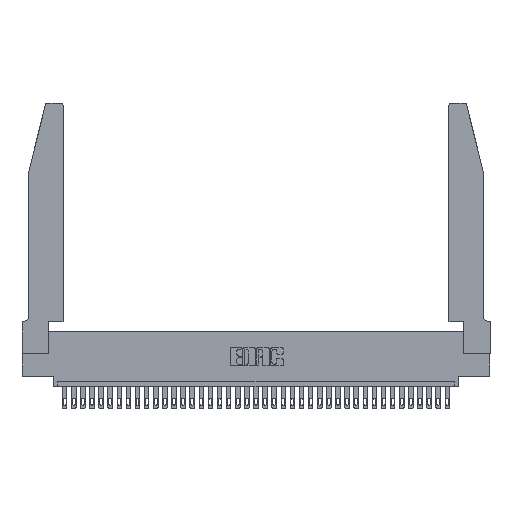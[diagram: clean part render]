
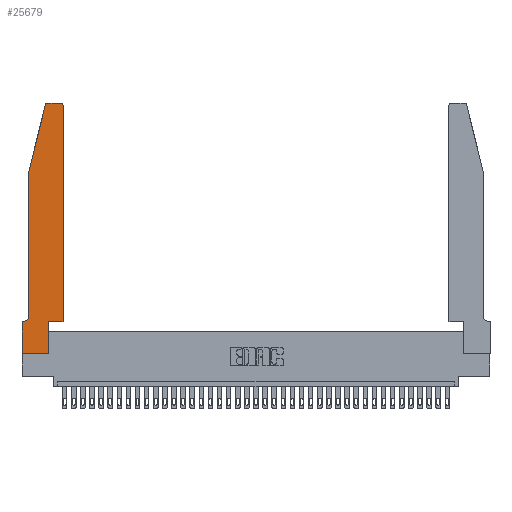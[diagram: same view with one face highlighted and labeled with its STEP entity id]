
A CAD part, top view. The second image highlights one B-rep face of the part: STEP entity #25679.
In plain terms, the highlighted planar face has unit normal (0, 0, 1).
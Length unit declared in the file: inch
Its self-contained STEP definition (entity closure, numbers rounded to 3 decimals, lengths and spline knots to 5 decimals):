
#149 = ORIENTED_EDGE ( 'NONE', *, *, #27881, .T. ) ;
#328 = VERTEX_POINT ( 'NONE', #6123 ) ;
#827 = LINE ( 'NONE', #27779, #32535 ) ;
#901 = EDGE_CURVE ( 'NONE', #5973, #25247, #16277, .T. ) ;
#1296 = CARTESIAN_POINT ( 'NONE',  ( 0., 0., 0.37 ) ) ;
#1358 = VERTEX_POINT ( 'NONE', #23213 ) ;
#1523 = CARTESIAN_POINT ( 'NONE',  ( 0.2865, 0.35, 0.37 ) ) ;
#1813 = ORIENTED_EDGE ( 'NONE', *, *, #10151, .T. ) ;
#2180 = ORIENTED_EDGE ( 'NONE', *, *, #6157, .T. ) ;
#2264 = CARTESIAN_POINT ( 'NONE',  ( 0.284, 2.72, 0.37 ) ) ;
#2333 = EDGE_CURVE ( 'NONE', #1358, #5973, #3722, .T. ) ;
#2733 = EDGE_CURVE ( 'NONE', #30739, #11146, #34075, .T. ) ;
#2929 = VERTEX_POINT ( 'NONE', #9198 ) ;
#2999 = VECTOR ( 'NONE', #15496, 39.37008 ) ;
#3722 = CIRCLE ( 'NONE', #23131, 0.07 ) ;
#3859 = FACE_OUTER_BOUND ( 'NONE', #23559, .T. ) ;
#4336 = CARTESIAN_POINT ( 'NONE',  ( 0., 0.35, 0.37 ) ) ;
#4540 = CARTESIAN_POINT ( 'NONE',  ( 0.25487, 2.72718, 0.37 ) ) ;
#4956 = CARTESIAN_POINT ( 'NONE',  ( 0.4505, 0.35, 0.37 ) ) ;
#5092 = DIRECTION ( 'NONE',  ( 1., 0., 0. ) ) ;
#5249 = LINE ( 'NONE', #1523, #2999 ) ;
#5566 = PLANE ( 'NONE',  #6493 ) ;
#5584 = VERTEX_POINT ( 'NONE', #31289 ) ;
#5973 = VERTEX_POINT ( 'NONE', #17368 ) ;
#6123 = CARTESIAN_POINT ( 'NONE',  ( 0., 0., 0.37 ) ) ;
#6157 = EDGE_CURVE ( 'NONE', #5584, #30739, #11033, .T. ) ;
#6173 = VECTOR ( 'NONE', #15835, 39.37008 ) ;
#6493 = AXIS2_PLACEMENT_3D ( 'NONE', #25360, #31089, #13894 ) ;
#6635 = DIRECTION ( 'NONE',  ( -1., 0., 0. ) ) ;
#6755 = EDGE_CURVE ( 'NONE', #11146, #10563, #12286, .T. ) ;
#7275 = EDGE_CURVE ( 'NONE', #328, #8594, #35431, .T. ) ;
#7518 = ORIENTED_EDGE ( 'NONE', *, *, #2733, .T. ) ;
#7609 = DIRECTION ( 'NONE',  ( -0.239, -0.971, 0. ) ) ;
#8113 = DIRECTION ( 'NONE',  ( 0., 0., 1. ) ) ;
#8195 = CARTESIAN_POINT ( 'NONE',  ( 0.2865, 0.35, 0.37 ) ) ;
#8306 = AXIS2_PLACEMENT_3D ( 'NONE', #16663, #22004, #5092 ) ;
#8594 = VERTEX_POINT ( 'NONE', #35665 ) ;
#9198 = CARTESIAN_POINT ( 'NONE',  ( 0.4505, 2.72, 0.37 ) ) ;
#9960 = VECTOR ( 'NONE', #32104, 39.37008 ) ;
#10151 = EDGE_CURVE ( 'NONE', #26637, #32149, #827, .T. ) ;
#10563 = VERTEX_POINT ( 'NONE', #15590 ) ;
#11033 = LINE ( 'NONE', #36269, #13682 ) ;
#11146 = VERTEX_POINT ( 'NONE', #4540 ) ;
#11243 = EDGE_CURVE ( 'NONE', #8594, #26637, #5249, .T. ) ;
#11865 = CARTESIAN_POINT ( 'NONE',  ( 0.0755, 0.35, 0.37 ) ) ;
#11964 = ORIENTED_EDGE ( 'NONE', *, *, #7275, .T. ) ;
#12286 = LINE ( 'NONE', #21658, #34613 ) ;
#12341 = CARTESIAN_POINT ( 'NONE',  ( 0.0755, 2., 0.37 ) ) ;
#12414 = ORIENTED_EDGE ( 'NONE', *, *, #2333, .T. ) ;
#12809 = CARTESIAN_POINT ( 'NONE',  ( 0.4505, 0.35, 0.37 ) ) ;
#13217 = EDGE_CURVE ( 'NONE', #10563, #1358, #33958, .T. ) ;
#13682 = VECTOR ( 'NONE', #15473, 39.37008 ) ;
#13785 = ORIENTED_EDGE ( 'NONE', *, *, #35846, .T. ) ;
#13894 = DIRECTION ( 'NONE',  ( 1., 0., 0. ) ) ;
#14136 = LINE ( 'NONE', #1296, #22592 ) ;
#15473 = DIRECTION ( 'NONE',  ( -1., 0., 0. ) ) ;
#15496 = DIRECTION ( 'NONE',  ( 0., 1., 0. ) ) ;
#15590 = CARTESIAN_POINT ( 'NONE',  ( 0.0755, 2., 0.37 ) ) ;
#15835 = DIRECTION ( 'NONE',  ( 0., -1., 0. ) ) ;
#16038 = AXIS2_PLACEMENT_3D ( 'NONE', #2264, #8113, #22303 ) ;
#16277 = LINE ( 'NONE', #11865, #31441 ) ;
#16663 = CARTESIAN_POINT ( 'NONE',  ( 0.4205, 2.72, 0.37 ) ) ;
#17368 = CARTESIAN_POINT ( 'NONE',  ( 0.0055, 0.35, 0.37 ) ) ;
#20556 = ORIENTED_EDGE ( 'NONE', *, *, #901, .T. ) ;
#20938 = EDGE_CURVE ( 'NONE', #25247, #328, #14136, .T. ) ;
#21658 = CARTESIAN_POINT ( 'NONE',  ( 0.0755, 2., 0.37 ) ) ;
#22004 = DIRECTION ( 'NONE',  ( 0., 0., 1. ) ) ;
#22303 = DIRECTION ( 'NONE',  ( 1., 0., 0. ) ) ;
#22393 = ORIENTED_EDGE ( 'NONE', *, *, #20938, .T. ) ;
#22592 = VECTOR ( 'NONE', #32202, 39.37008 ) ;
#23131 = AXIS2_PLACEMENT_3D ( 'NONE', #23674, #24041, #26917 ) ;
#23213 = CARTESIAN_POINT ( 'NONE',  ( 0.0755, 0.42, 0.37 ) ) ;
#23559 = EDGE_LOOP ( 'NONE', ( #2180, #7518, #34823, #26884, #12414, #20556, #22393, #11964, #29960, #1813, #149, #13785 ) ) ;
#23674 = CARTESIAN_POINT ( 'NONE',  ( 0.0055, 0.42, 0.37 ) ) ;
#24018 = DIRECTION ( 'NONE',  ( 0., 1., 0. ) ) ;
#24041 = DIRECTION ( 'NONE',  ( 0., 0., -1. ) ) ;
#25247 = VERTEX_POINT ( 'NONE', #4336 ) ;
#25360 = CARTESIAN_POINT ( 'NONE',  ( 0., 0.35, 0.37 ) ) ;
#25679 = ADVANCED_FACE ( 'NONE', ( #3859 ), #5566, .T. ) ;
#26637 = VERTEX_POINT ( 'NONE', #8195 ) ;
#26884 = ORIENTED_EDGE ( 'NONE', *, *, #13217, .T. ) ;
#26917 = DIRECTION ( 'NONE',  ( -1., 0., 0. ) ) ;
#27279 = LINE ( 'NONE', #12809, #29522 ) ;
#27779 = CARTESIAN_POINT ( 'NONE',  ( 0.4505, 0.35, 0.37 ) ) ;
#27798 = CARTESIAN_POINT ( 'NONE',  ( 0., 0., 0.37 ) ) ;
#27881 = EDGE_CURVE ( 'NONE', #32149, #2929, #27279, .T. ) ;
#29164 = CARTESIAN_POINT ( 'NONE',  ( 0.284, 2.75, 0.37 ) ) ;
#29485 = CIRCLE ( 'NONE', #8306, 0.03 ) ;
#29522 = VECTOR ( 'NONE', #24018, 39.37008 ) ;
#29960 = ORIENTED_EDGE ( 'NONE', *, *, #11243, .T. ) ;
#30674 = DIRECTION ( 'NONE',  ( 1., 0., 0. ) ) ;
#30739 = VERTEX_POINT ( 'NONE', #29164 ) ;
#31089 = DIRECTION ( 'NONE',  ( 0., 0., 1. ) ) ;
#31289 = CARTESIAN_POINT ( 'NONE',  ( 0.4205, 2.75, 0.37 ) ) ;
#31441 = VECTOR ( 'NONE', #6635, 39.37008 ) ;
#32104 = DIRECTION ( 'NONE',  ( 1., 0., 0. ) ) ;
#32149 = VERTEX_POINT ( 'NONE', #4956 ) ;
#32202 = DIRECTION ( 'NONE',  ( 0., -1., 0. ) ) ;
#32535 = VECTOR ( 'NONE', #30674, 39.37008 ) ;
#33958 = LINE ( 'NONE', #12341, #6173 ) ;
#34075 = CIRCLE ( 'NONE', #16038, 0.03 ) ;
#34613 = VECTOR ( 'NONE', #7609, 39.37008 ) ;
#34823 = ORIENTED_EDGE ( 'NONE', *, *, #6755, .T. ) ;
#35431 = LINE ( 'NONE', #27798, #9960 ) ;
#35665 = CARTESIAN_POINT ( 'NONE',  ( 0.2865, 0., 0.37 ) ) ;
#35846 = EDGE_CURVE ( 'NONE', #2929, #5584, #29485, .T. ) ;
#36269 = CARTESIAN_POINT ( 'NONE',  ( 0.2605, 2.75, 0.37 ) ) ;
